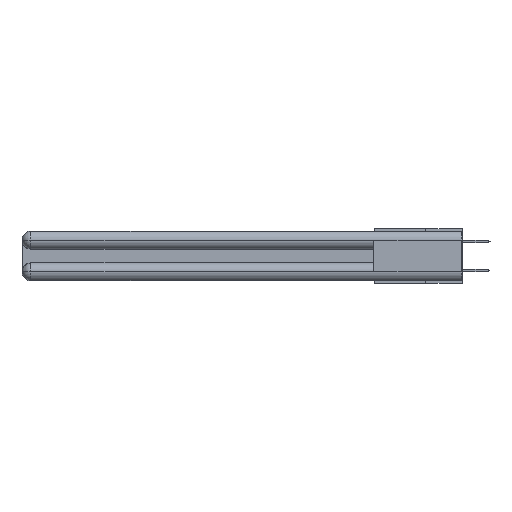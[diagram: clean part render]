
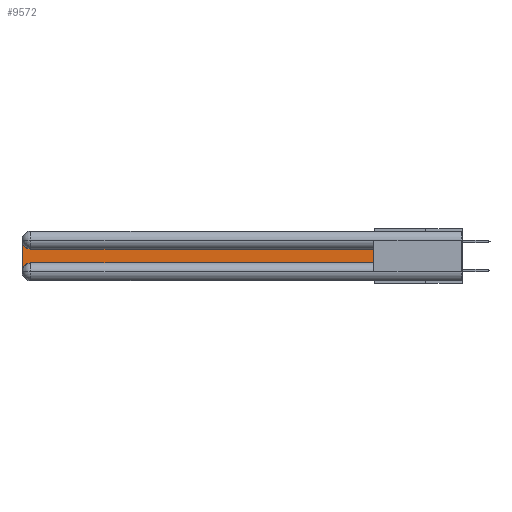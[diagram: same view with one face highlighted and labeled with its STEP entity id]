
A CAD part, left-side view. The second image highlights one B-rep face of the part: STEP entity #9572.
In plain terms, the highlighted planar face has unit normal (-1, 0, 0).
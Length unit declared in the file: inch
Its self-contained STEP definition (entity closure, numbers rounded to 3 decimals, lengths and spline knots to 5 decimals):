
#1152 = CARTESIAN_POINT ( 'NONE',  ( 0.075, 3., -0.0625 ) ) ;
#3346 = EDGE_CURVE ( 'NONE', #29672, #27962, #23596, .T. ) ;
#4237 = LINE ( 'NONE', #26580, #30368 ) ;
#4851 = VECTOR ( 'NONE', #5604, 39.37008 ) ;
#4965 = VERTEX_POINT ( 'NONE', #23534 ) ;
#5527 = DIRECTION ( 'NONE',  ( 1., 0., 0. ) ) ;
#5539 = CARTESIAN_POINT ( 'NONE',  ( 0.075, 3., -0.1225 ) ) ;
#5604 = DIRECTION ( 'NONE',  ( 0., -1., 0. ) ) ;
#7033 = ORIENTED_EDGE ( 'NONE', *, *, #10890, .T. ) ;
#7486 = VECTOR ( 'NONE', #30644, 39.37008 ) ;
#7650 = DIRECTION ( 'NONE',  ( 0., 0., -1. ) ) ;
#7864 = CARTESIAN_POINT ( 'NONE',  ( 0.075, 2.94, -0.0625 ) ) ;
#8072 = DIRECTION ( 'NONE',  ( 0., 0., -1. ) ) ;
#8530 = EDGE_CURVE ( 'NONE', #17857, #29672, #21768, .T. ) ;
#8962 = DIRECTION ( 'NONE',  ( 0., 0., -1. ) ) ;
#9550 = CARTESIAN_POINT ( 'NONE',  ( 0.075, 0.6, -0.2175 ) ) ;
#9572 = ADVANCED_FACE ( 'NONE', ( #19611 ), #30013, .F. ) ;
#9933 = CARTESIAN_POINT ( 'NONE',  ( 0.075, 2.94, -0.2775 ) ) ;
#10890 = EDGE_CURVE ( 'NONE', #4965, #17857, #20299, .T. ) ;
#12440 = DIRECTION ( 'NONE',  ( 0., 0., -1. ) ) ;
#12599 = DIRECTION ( 'NONE',  ( 1., 0., 0. ) ) ;
#13724 = ORIENTED_EDGE ( 'NONE', *, *, #30561, .T. ) ;
#15800 = CARTESIAN_POINT ( 'NONE',  ( 0.075, 0.6, -0.2175 ) ) ;
#16179 = CARTESIAN_POINT ( 'NONE',  ( 0.075, 3., -0.2775 ) ) ;
#16779 = CIRCLE ( 'NONE', #18482, 0.06 ) ;
#17857 = VERTEX_POINT ( 'NONE', #9550 ) ;
#18482 = AXIS2_PLACEMENT_3D ( 'NONE', #9933, #22346, #12440 ) ;
#19611 = FACE_OUTER_BOUND ( 'NONE', #20797, .T. ) ;
#19715 = CARTESIAN_POINT ( 'NONE',  ( 0.075, 2.94, -0.1225 ) ) ;
#20299 = LINE ( 'NONE', #15800, #4851 ) ;
#20797 = EDGE_LOOP ( 'NONE', ( #22304, #27381, #22149, #13724, #7033, #30081 ) ) ;
#21768 = LINE ( 'NONE', #28226, #7486 ) ;
#22149 = ORIENTED_EDGE ( 'NONE', *, *, #26267, .T. ) ;
#22304 = ORIENTED_EDGE ( 'NONE', *, *, #3346, .T. ) ;
#22346 = DIRECTION ( 'NONE',  ( 1., 0., 0. ) ) ;
#22854 = AXIS2_PLACEMENT_3D ( 'NONE', #7864, #5527, #8072 ) ;
#23534 = CARTESIAN_POINT ( 'NONE',  ( 0.075, 2.94, -0.2175 ) ) ;
#23596 = LINE ( 'NONE', #29407, #31913 ) ;
#24669 = EDGE_CURVE ( 'NONE', #27962, #28569, #30050, .T. ) ;
#26108 = CARTESIAN_POINT ( 'NONE',  ( 0.075, 0.6, -0.1225 ) ) ;
#26267 = EDGE_CURVE ( 'NONE', #28569, #27914, #4237, .T. ) ;
#26580 = CARTESIAN_POINT ( 'NONE',  ( 0.075, 3., -0.2175 ) ) ;
#27381 = ORIENTED_EDGE ( 'NONE', *, *, #24669, .T. ) ;
#27914 = VERTEX_POINT ( 'NONE', #16179 ) ;
#27962 = VERTEX_POINT ( 'NONE', #19715 ) ;
#28226 = CARTESIAN_POINT ( 'NONE',  ( 0.075, 0.6, -0.2175 ) ) ;
#28569 = VERTEX_POINT ( 'NONE', #1152 ) ;
#28790 = AXIS2_PLACEMENT_3D ( 'NONE', #5539, #12599, #7650 ) ;
#29407 = CARTESIAN_POINT ( 'NONE',  ( 0.075, 0.6, -0.1225 ) ) ;
#29672 = VERTEX_POINT ( 'NONE', #26108 ) ;
#30013 = PLANE ( 'NONE',  #28790 ) ;
#30050 = CIRCLE ( 'NONE', #22854, 0.06 ) ;
#30081 = ORIENTED_EDGE ( 'NONE', *, *, #8530, .T. ) ;
#30368 = VECTOR ( 'NONE', #8962, 39.37008 ) ;
#30561 = EDGE_CURVE ( 'NONE', #27914, #4965, #16779, .T. ) ;
#30644 = DIRECTION ( 'NONE',  ( 0., 0., 1. ) ) ;
#31913 = VECTOR ( 'NONE', #32173, 39.37008 ) ;
#32173 = DIRECTION ( 'NONE',  ( 0., 1., 0. ) ) ;
